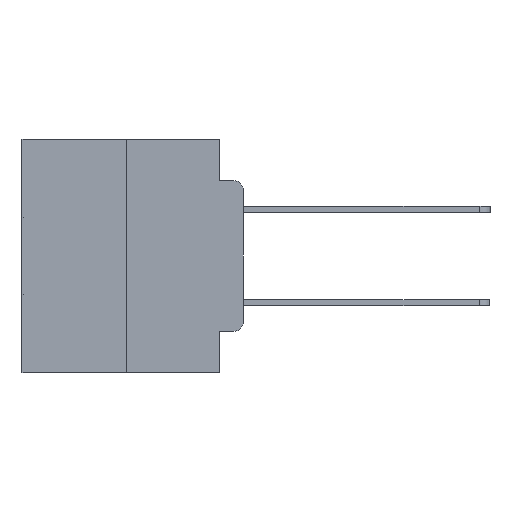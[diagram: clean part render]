
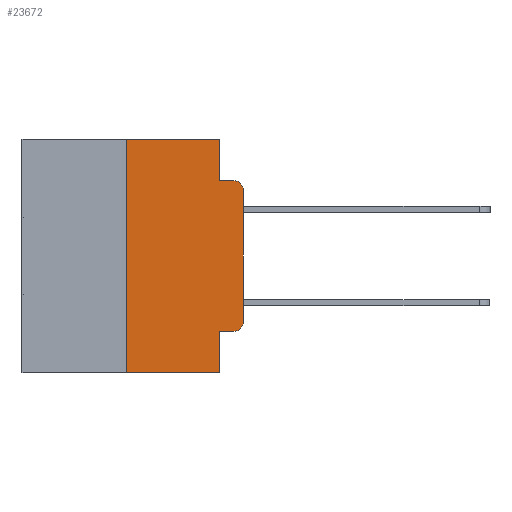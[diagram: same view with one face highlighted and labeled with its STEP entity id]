
A CAD part, left-side view. The second image highlights one B-rep face of the part: STEP entity #23672.
In plain terms, the highlighted planar face has unit normal (-1, 0, 0).
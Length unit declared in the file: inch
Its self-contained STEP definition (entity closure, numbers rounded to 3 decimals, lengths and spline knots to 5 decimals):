
#351 = CARTESIAN_POINT ( 'NONE',  ( 0., 0.051, -0.5 ) ) ;
#758 = CARTESIAN_POINT ( 'NONE',  ( 0., 0.02, -0.4115 ) ) ;
#1308 = ORIENTED_EDGE ( 'NONE', *, *, #23856, .T. ) ;
#1476 = LINE ( 'NONE', #20819, #13450 ) ;
#1537 = EDGE_CURVE ( 'NONE', #9624, #22713, #1476, .T. ) ;
#1911 = CARTESIAN_POINT ( 'NONE',  ( 0., 0.02, -0.0885 ) ) ;
#2243 = ORIENTED_EDGE ( 'NONE', *, *, #8829, .F. ) ;
#2336 = VERTEX_POINT ( 'NONE', #18310 ) ;
#2604 = ORIENTED_EDGE ( 'NONE', *, *, #8807, .F. ) ;
#2808 = DIRECTION ( 'NONE',  ( 0., -1., 0. ) ) ;
#2866 = LINE ( 'NONE', #17347, #8188 ) ;
#3297 = ORIENTED_EDGE ( 'NONE', *, *, #11259, .T. ) ;
#3498 = CARTESIAN_POINT ( 'NONE',  ( 0., 0.051, -0.0885 ) ) ;
#3589 = ORIENTED_EDGE ( 'NONE', *, *, #14777, .T. ) ;
#3842 = LINE ( 'NONE', #27840, #20800 ) ;
#4624 = DIRECTION ( 'NONE',  ( 0., -1., 0. ) ) ;
#4818 = LINE ( 'NONE', #17854, #10066 ) ;
#5230 = VERTEX_POINT ( 'NONE', #26508 ) ;
#5603 = CARTESIAN_POINT ( 'NONE',  ( 0., 0.25, 0. ) ) ;
#5754 = DIRECTION ( 'NONE',  ( 0., -1., 0. ) ) ;
#5812 = ORIENTED_EDGE ( 'NONE', *, *, #1537, .F. ) ;
#5817 = EDGE_CURVE ( 'NONE', #22713, #7230, #16617, .T. ) ;
#5872 = ORIENTED_EDGE ( 'NONE', *, *, #24435, .T. ) ;
#6196 = DIRECTION ( 'NONE',  ( 0., 0., -1. ) ) ;
#6493 = LINE ( 'NONE', #3498, #17528 ) ;
#6947 = ORIENTED_EDGE ( 'NONE', *, *, #7361, .F. ) ;
#7211 = CARTESIAN_POINT ( 'NONE',  ( 0., 0.02, -0.3915 ) ) ;
#7230 = VERTEX_POINT ( 'NONE', #9888 ) ;
#7332 = VERTEX_POINT ( 'NONE', #1911 ) ;
#7361 = EDGE_CURVE ( 'NONE', #7230, #7332, #6493, .T. ) ;
#8052 = ORIENTED_EDGE ( 'NONE', *, *, #5817, .F. ) ;
#8188 = VECTOR ( 'NONE', #8633, 39.37008 ) ;
#8633 = DIRECTION ( 'NONE',  ( 0., 0., -1. ) ) ;
#8807 = EDGE_CURVE ( 'NONE', #2336, #9624, #26214, .T. ) ;
#8829 = EDGE_CURVE ( 'NONE', #25735, #15078, #2866, .T. ) ;
#9445 = DIRECTION ( 'NONE',  ( 0., 0., -1. ) ) ;
#9487 = CARTESIAN_POINT ( 'NONE',  ( 0., 0.051, 0. ) ) ;
#9624 = VERTEX_POINT ( 'NONE', #5603 ) ;
#9840 = CARTESIAN_POINT ( 'NONE',  ( 0., 0.02, -0.1085 ) ) ;
#9888 = CARTESIAN_POINT ( 'NONE',  ( 0., 0.051, -0.0885 ) ) ;
#10066 = VECTOR ( 'NONE', #4624, 39.37008 ) ;
#10170 = CARTESIAN_POINT ( 'NONE',  ( 0., 0., -0.3915 ) ) ;
#10500 = CARTESIAN_POINT ( 'NONE',  ( 0., 0.473, 0. ) ) ;
#11128 = FACE_OUTER_BOUND ( 'NONE', #25112, .T. ) ;
#11259 = EDGE_CURVE ( 'NONE', #12723, #14670, #24287, .T. ) ;
#11674 = CIRCLE ( 'NONE', #28307, 0.02 ) ;
#12044 = DIRECTION ( 'NONE',  ( 0., 0., -1. ) ) ;
#12723 = VERTEX_POINT ( 'NONE', #758 ) ;
#12888 = DIRECTION ( 'NONE',  ( 0., 0., 1. ) ) ;
#13450 = VECTOR ( 'NONE', #16311, 39.37008 ) ;
#14670 = VERTEX_POINT ( 'NONE', #10170 ) ;
#14777 = EDGE_CURVE ( 'NONE', #14670, #5230, #3842, .T. ) ;
#15078 = VERTEX_POINT ( 'NONE', #351 ) ;
#15952 = CARTESIAN_POINT ( 'NONE',  ( 0., 0.051, 0. ) ) ;
#16311 = DIRECTION ( 'NONE',  ( 0., -1., 0. ) ) ;
#16617 = LINE ( 'NONE', #15952, #22408 ) ;
#17192 = PLANE ( 'NONE',  #19173 ) ;
#17347 = CARTESIAN_POINT ( 'NONE',  ( 0., 0.051, 0. ) ) ;
#17528 = VECTOR ( 'NONE', #5754, 39.37008 ) ;
#17854 = CARTESIAN_POINT ( 'NONE',  ( 0., 0.051, -0.4115 ) ) ;
#18310 = CARTESIAN_POINT ( 'NONE',  ( 0., 0.25, -0.5 ) ) ;
#18339 = CARTESIAN_POINT ( 'NONE',  ( 0., 0.473, -0.5 ) ) ;
#19173 = AXIS2_PLACEMENT_3D ( 'NONE', #10500, #19414, #6196 ) ;
#19414 = DIRECTION ( 'NONE',  ( 1., 0., 0. ) ) ;
#19487 = CARTESIAN_POINT ( 'NONE',  ( 0., 0.25, 0. ) ) ;
#20800 = VECTOR ( 'NONE', #25651, 39.37008 ) ;
#20819 = CARTESIAN_POINT ( 'NONE',  ( 0., 0.473, 0. ) ) ;
#21245 = VECTOR ( 'NONE', #12888, 39.37008 ) ;
#21865 = ORIENTED_EDGE ( 'NONE', *, *, #25796, .T. ) ;
#22408 = VECTOR ( 'NONE', #26669, 39.37008 ) ;
#22543 = DIRECTION ( 'NONE',  ( -1., 0., 0. ) ) ;
#22684 = VECTOR ( 'NONE', #2808, 39.37008 ) ;
#22713 = VERTEX_POINT ( 'NONE', #9487 ) ;
#23672 = ADVANCED_FACE ( 'NONE', ( #11128 ), #17192, .F. ) ;
#23856 = EDGE_CURVE ( 'NONE', #25735, #12723, #4818, .T. ) ;
#24287 = CIRCLE ( 'NONE', #24890, 0.02 ) ;
#24435 = EDGE_CURVE ( 'NONE', #2336, #15078, #28289, .T. ) ;
#24789 = CARTESIAN_POINT ( 'NONE',  ( 0., 0.051, -0.4115 ) ) ;
#24890 = AXIS2_PLACEMENT_3D ( 'NONE', #7211, #22543, #9445 ) ;
#25053 = DIRECTION ( 'NONE',  ( -1., 0., 0. ) ) ;
#25112 = EDGE_LOOP ( 'NONE', ( #3589, #21865, #6947, #8052, #5812, #2604, #5872, #2243, #1308, #3297 ) ) ;
#25651 = DIRECTION ( 'NONE',  ( 0., 0., 1. ) ) ;
#25735 = VERTEX_POINT ( 'NONE', #24789 ) ;
#25796 = EDGE_CURVE ( 'NONE', #5230, #7332, #11674, .T. ) ;
#26214 = LINE ( 'NONE', #19487, #21245 ) ;
#26508 = CARTESIAN_POINT ( 'NONE',  ( 0., 0., -0.1085 ) ) ;
#26669 = DIRECTION ( 'NONE',  ( 0., 0., -1. ) ) ;
#27840 = CARTESIAN_POINT ( 'NONE',  ( 0., 0., 0. ) ) ;
#28289 = LINE ( 'NONE', #18339, #22684 ) ;
#28307 = AXIS2_PLACEMENT_3D ( 'NONE', #9840, #25053, #12044 ) ;
